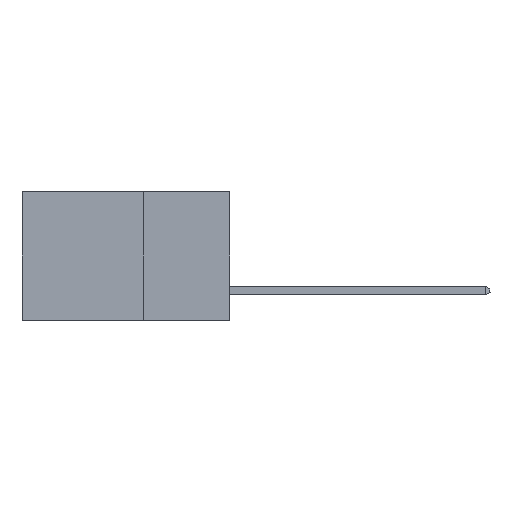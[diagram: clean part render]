
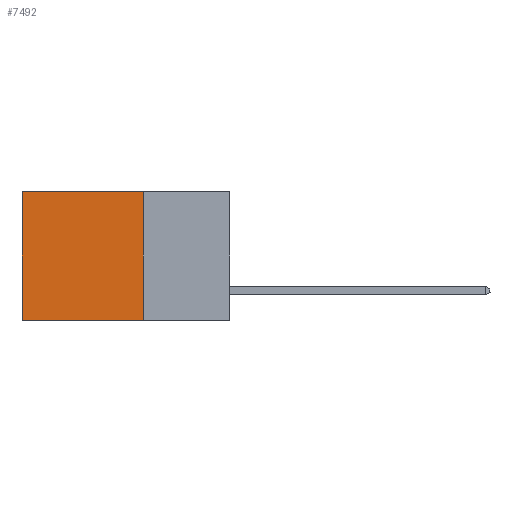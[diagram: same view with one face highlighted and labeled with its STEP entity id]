
A CAD part, left-side view. The second image highlights one B-rep face of the part: STEP entity #7492.
In plain terms, the highlighted planar face has unit normal (-1, 0, 0).
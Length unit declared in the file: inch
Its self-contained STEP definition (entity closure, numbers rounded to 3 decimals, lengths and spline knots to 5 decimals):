
#232 = VECTOR ( 'NONE', #1948, 39.37008 ) ;
#873 = DIRECTION ( 'NONE',  ( 1., 0., 0. ) ) ;
#1409 = VERTEX_POINT ( 'NONE', #14844 ) ;
#1816 = VERTEX_POINT ( 'NONE', #8879 ) ;
#1948 = DIRECTION ( 'NONE',  ( 0., 0., -1. ) ) ;
#2244 = EDGE_CURVE ( 'NONE', #3639, #16323, #6108, .T. ) ;
#2907 = CARTESIAN_POINT ( 'NONE',  ( 0.298, 0.6, 0. ) ) ;
#3160 = VECTOR ( 'NONE', #7780, 39.37008 ) ;
#3639 = VERTEX_POINT ( 'NONE', #11837 ) ;
#4312 = LINE ( 'NONE', #7442, #12532 ) ;
#4502 = AXIS2_PLACEMENT_3D ( 'NONE', #8785, #873, #10027 ) ;
#4656 = DIRECTION ( 'NONE',  ( 0., 0., -1. ) ) ;
#4697 = FACE_OUTER_BOUND ( 'NONE', #13620, .T. ) ;
#4987 = DIRECTION ( 'NONE',  ( 0., 1., 0. ) ) ;
#5653 = LINE ( 'NONE', #16290, #14898 ) ;
#5783 = ORIENTED_EDGE ( 'NONE', *, *, #12893, .F. ) ;
#5805 = LINE ( 'NONE', #12431, #232 ) ;
#6108 = LINE ( 'NONE', #14348, #3160 ) ;
#6248 = EDGE_CURVE ( 'NONE', #1816, #1409, #4312, .T. ) ;
#6289 = PLANE ( 'NONE',  #4502 ) ;
#7442 = CARTESIAN_POINT ( 'NONE',  ( 0.298, 0.25, -0.37 ) ) ;
#7492 = ADVANCED_FACE ( 'NONE', ( #4697 ), #6289, .F. ) ;
#7780 = DIRECTION ( 'NONE',  ( 0., 1., 0. ) ) ;
#8785 = CARTESIAN_POINT ( 'NONE',  ( 0.298, 0.25, 0. ) ) ;
#8879 = CARTESIAN_POINT ( 'NONE',  ( 0.298, 0.25, -0.37 ) ) ;
#9139 = ORIENTED_EDGE ( 'NONE', *, *, #6248, .F. ) ;
#10027 = DIRECTION ( 'NONE',  ( 0., 0., -1. ) ) ;
#11837 = CARTESIAN_POINT ( 'NONE',  ( 0.298, 0.25, 0. ) ) ;
#12431 = CARTESIAN_POINT ( 'NONE',  ( 0.298, 0.6, 0. ) ) ;
#12532 = VECTOR ( 'NONE', #4987, 39.37008 ) ;
#12893 = EDGE_CURVE ( 'NONE', #3639, #1816, #5653, .T. ) ;
#13620 = EDGE_LOOP ( 'NONE', ( #13726, #9139, #5783, #14756 ) ) ;
#13726 = ORIENTED_EDGE ( 'NONE', *, *, #14607, .T. ) ;
#14348 = CARTESIAN_POINT ( 'NONE',  ( 0.298, 0.25, 0. ) ) ;
#14607 = EDGE_CURVE ( 'NONE', #16323, #1409, #5805, .T. ) ;
#14756 = ORIENTED_EDGE ( 'NONE', *, *, #2244, .T. ) ;
#14844 = CARTESIAN_POINT ( 'NONE',  ( 0.298, 0.6, -0.37 ) ) ;
#14898 = VECTOR ( 'NONE', #4656, 39.37008 ) ;
#16290 = CARTESIAN_POINT ( 'NONE',  ( 0.298, 0.25, 0. ) ) ;
#16323 = VERTEX_POINT ( 'NONE', #2907 ) ;
